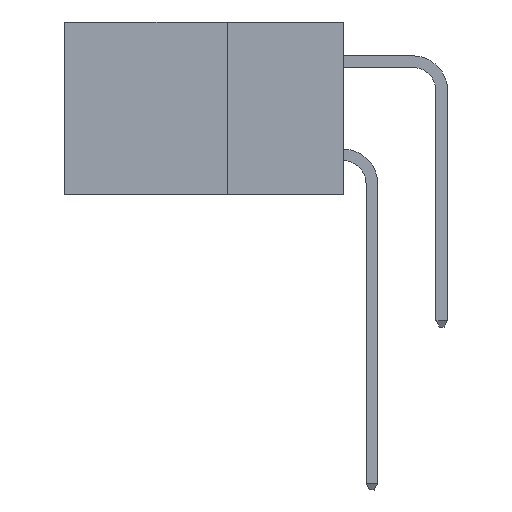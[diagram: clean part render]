
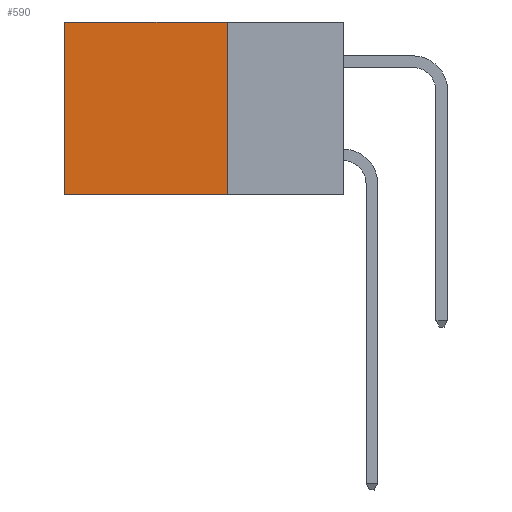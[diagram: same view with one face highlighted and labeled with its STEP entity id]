
A CAD part, left-side view. The second image highlights one B-rep face of the part: STEP entity #590.
In plain terms, the highlighted planar face has unit normal (-1, 0, 0).
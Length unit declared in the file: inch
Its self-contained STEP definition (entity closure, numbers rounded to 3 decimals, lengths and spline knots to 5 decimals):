
#360 = CARTESIAN_POINT ( 'NONE',  ( 0.298, 0.6, 0. ) ) ;
#590 = ADVANCED_FACE ( 'NONE', ( #11875 ), #14672, .F. ) ;
#884 = EDGE_CURVE ( 'NONE', #8619, #7354, #11690, .T. ) ;
#2219 = VECTOR ( 'NONE', #11492, 39.37008 ) ;
#2253 = CARTESIAN_POINT ( 'NONE',  ( 0.298, 0.25, 0. ) ) ;
#2303 = DIRECTION ( 'NONE',  ( 1., 0., 0. ) ) ;
#2696 = DIRECTION ( 'NONE',  ( 0., 0., -1. ) ) ;
#2859 = ORIENTED_EDGE ( 'NONE', *, *, #3300, .F. ) ;
#3300 = EDGE_CURVE ( 'NONE', #3932, #6626, #16056, .T. ) ;
#3318 = VECTOR ( 'NONE', #2696, 39.37008 ) ;
#3625 = DIRECTION ( 'NONE',  ( 0., 0., -1. ) ) ;
#3932 = VERTEX_POINT ( 'NONE', #14209 ) ;
#4344 = ORIENTED_EDGE ( 'NONE', *, *, #14430, .F. ) ;
#5320 = CARTESIAN_POINT ( 'NONE',  ( 0.298, 0.6, -0.37 ) ) ;
#5901 = VECTOR ( 'NONE', #3625, 39.37008 ) ;
#5926 = ORIENTED_EDGE ( 'NONE', *, *, #884, .T. ) ;
#6626 = VERTEX_POINT ( 'NONE', #5320 ) ;
#7205 = VECTOR ( 'NONE', #11024, 39.37008 ) ;
#7354 = VERTEX_POINT ( 'NONE', #12710 ) ;
#8002 = EDGE_LOOP ( 'NONE', ( #14654, #2859, #4344, #5926 ) ) ;
#8619 = VERTEX_POINT ( 'NONE', #11836 ) ;
#9858 = CARTESIAN_POINT ( 'NONE',  ( 0.298, 0.25, -0.37 ) ) ;
#9896 = CARTESIAN_POINT ( 'NONE',  ( 0.298, 0.25, 0. ) ) ;
#10600 = EDGE_CURVE ( 'NONE', #7354, #6626, #12946, .T. ) ;
#11024 = DIRECTION ( 'NONE',  ( 0., 1., 0. ) ) ;
#11492 = DIRECTION ( 'NONE',  ( 0., 1., 0. ) ) ;
#11606 = CARTESIAN_POINT ( 'NONE',  ( 0.298, 0.25, 0. ) ) ;
#11690 = LINE ( 'NONE', #11606, #2219 ) ;
#11836 = CARTESIAN_POINT ( 'NONE',  ( 0.298, 0.25, 0. ) ) ;
#11875 = FACE_OUTER_BOUND ( 'NONE', #8002, .T. ) ;
#12125 = AXIS2_PLACEMENT_3D ( 'NONE', #2253, #2303, #15939 ) ;
#12710 = CARTESIAN_POINT ( 'NONE',  ( 0.298, 0.6, 0. ) ) ;
#12946 = LINE ( 'NONE', #360, #3318 ) ;
#14209 = CARTESIAN_POINT ( 'NONE',  ( 0.298, 0.25, -0.37 ) ) ;
#14430 = EDGE_CURVE ( 'NONE', #8619, #3932, #14598, .T. ) ;
#14598 = LINE ( 'NONE', #9896, #5901 ) ;
#14654 = ORIENTED_EDGE ( 'NONE', *, *, #10600, .T. ) ;
#14672 = PLANE ( 'NONE',  #12125 ) ;
#15939 = DIRECTION ( 'NONE',  ( 0., 0., -1. ) ) ;
#16056 = LINE ( 'NONE', #9858, #7205 ) ;
